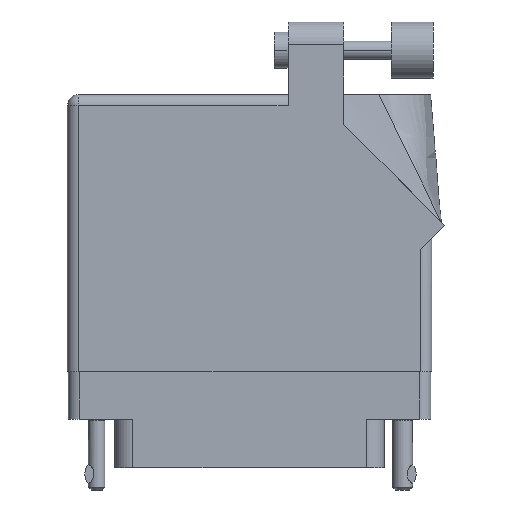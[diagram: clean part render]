
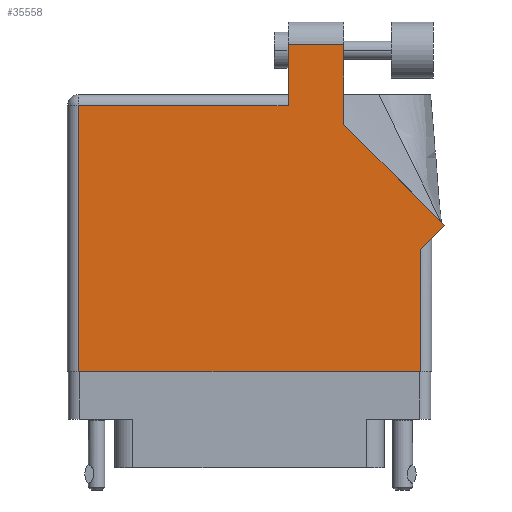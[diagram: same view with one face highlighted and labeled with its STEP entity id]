
A CAD part, front view. The second image highlights one B-rep face of the part: STEP entity #35558.
In plain terms, the highlighted face is planar.
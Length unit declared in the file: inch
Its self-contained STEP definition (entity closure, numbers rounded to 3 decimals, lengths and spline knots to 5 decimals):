
#1237 = EDGE_CURVE ( 'NONE', #14400, #40537, #26555, .T. ) ;
#1443 = CARTESIAN_POINT ( 'NONE',  ( 0., 1.468, 0. ) ) ;
#2325 = VECTOR ( 'NONE', #35104, 39.37008 ) ;
#3717 = VERTEX_POINT ( 'NONE', #31275 ) ;
#4277 = CARTESIAN_POINT ( 'NONE',  ( 1.217, 1.468, 0. ) ) ;
#5003 = EDGE_CURVE ( 'NONE', #3717, #17472, #18314, .T. ) ;
#5214 = CARTESIAN_POINT ( 'NONE',  ( 2.01, 0.737, 0. ) ) ;
#5677 = VECTOR ( 'NONE', #8949, 39.37008 ) ;
#5948 = CARTESIAN_POINT ( 'NONE',  ( 1.948, 0.737, 0. ) ) ;
#6201 = DIRECTION ( 'NONE',  ( 0., -1., 0. ) ) ;
#6716 = ORIENTED_EDGE ( 'NONE', *, *, #5003, .T. ) ;
#7235 = CARTESIAN_POINT ( 'NONE',  ( 2.08071, 0.80771, 0. ) ) ;
#8949 = DIRECTION ( 'NONE',  ( -1., 0., 0. ) ) ;
#9082 = DIRECTION ( 'NONE',  ( 1., 0., 0. ) ) ;
#9461 = ORIENTED_EDGE ( 'NONE', *, *, #38075, .T. ) ;
#9899 = VECTOR ( 'NONE', #6201, 39.37008 ) ;
#10427 = CARTESIAN_POINT ( 'NONE',  ( 0.062, 0., 0. ) ) ;
#10512 = LINE ( 'NONE', #5214, #2325 ) ;
#10582 = CARTESIAN_POINT ( 'NONE',  ( 1.524, 1.36442, 0. ) ) ;
#11581 = VERTEX_POINT ( 'NONE', #33478 ) ;
#11843 = CARTESIAN_POINT ( 'NONE',  ( 1.217, 1.805, 0. ) ) ;
#12568 = LINE ( 'NONE', #19613, #28801 ) ;
#12600 = ORIENTED_EDGE ( 'NONE', *, *, #44151, .T. ) ;
#13975 = ORIENTED_EDGE ( 'NONE', *, *, #20043, .T. ) ;
#14283 = VECTOR ( 'NONE', #41070, 39.37008 ) ;
#14400 = VERTEX_POINT ( 'NONE', #33937 ) ;
#14546 = ORIENTED_EDGE ( 'NONE', *, *, #37458, .T. ) ;
#14569 = ORIENTED_EDGE ( 'NONE', *, *, #42287, .T. ) ;
#14873 = DIRECTION ( 'NONE',  ( 0., 0., -1. ) ) ;
#15095 = LINE ( 'NONE', #24194, #9899 ) ;
#15404 = DIRECTION ( 'NONE',  ( 0., 1., 0. ) ) ;
#16024 = DIRECTION ( 'NONE',  ( -1., 0., 0. ) ) ;
#17309 = DIRECTION ( 'NONE',  ( 0., 1., 0. ) ) ;
#17425 = VECTOR ( 'NONE', #15404, 39.37008 ) ;
#17472 = VERTEX_POINT ( 'NONE', #34454 ) ;
#18314 = LINE ( 'NONE', #31293, #31669 ) ;
#19613 = CARTESIAN_POINT ( 'NONE',  ( 1.217, 1.805, 0. ) ) ;
#20043 = EDGE_CURVE ( 'NONE', #17472, #40275, #34700, .T. ) ;
#20277 = ORIENTED_EDGE ( 'NONE', *, *, #37798, .T. ) ;
#22317 = DIRECTION ( 'NONE',  ( -0.707, 0.707, 0. ) ) ;
#23098 = DIRECTION ( 'NONE',  ( -1., 0., 0. ) ) ;
#23368 = CARTESIAN_POINT ( 'NONE',  ( 1.948, 0.675, 0. ) ) ;
#23609 = VECTOR ( 'NONE', #22317, 39.37008 ) ;
#24194 = CARTESIAN_POINT ( 'NONE',  ( 1.217, 1.53, 0. ) ) ;
#25384 = VECTOR ( 'NONE', #17309, 39.37008 ) ;
#26555 = LINE ( 'NONE', #7235, #23609 ) ;
#27010 = VERTEX_POINT ( 'NONE', #11843 ) ;
#28801 = VECTOR ( 'NONE', #16024, 39.37008 ) ;
#29156 = FACE_OUTER_BOUND ( 'NONE', #36022, .T. ) ;
#29655 = CARTESIAN_POINT ( 'NONE',  ( 0., 1.53, 0. ) ) ;
#31275 = CARTESIAN_POINT ( 'NONE',  ( 0.062, 0., 0. ) ) ;
#31293 = CARTESIAN_POINT ( 'NONE',  ( 0., 0., 0. ) ) ;
#31669 = VECTOR ( 'NONE', #9082, 39.37008 ) ;
#31836 = AXIS2_PLACEMENT_3D ( 'NONE', #29655, #14873, #23098 ) ;
#32410 = LINE ( 'NONE', #1443, #5677 ) ;
#32449 = VERTEX_POINT ( 'NONE', #40043 ) ;
#33431 = CARTESIAN_POINT ( 'NONE',  ( 1.524, 1.36442, 0. ) ) ;
#33478 = CARTESIAN_POINT ( 'NONE',  ( 1.524, 1.805, 0. ) ) ;
#33937 = CARTESIAN_POINT ( 'NONE',  ( 2.08071, 0.80771, 0. ) ) ;
#34007 = LINE ( 'NONE', #10427, #14283 ) ;
#34454 = CARTESIAN_POINT ( 'NONE',  ( 1.948, 0., 0. ) ) ;
#34700 = LINE ( 'NONE', #5948, #25384 ) ;
#35104 = DIRECTION ( 'NONE',  ( 0.707, 0.707, 0. ) ) ;
#35558 = ADVANCED_FACE ( 'NONE', ( #29156 ), #44267, .F. ) ;
#36022 = EDGE_LOOP ( 'NONE', ( #20277, #38280, #9461, #14569, #12600, #6716, #13975, #14546, #42615 ) ) ;
#37458 = EDGE_CURVE ( 'NONE', #40275, #14400, #10512, .T. ) ;
#37798 = EDGE_CURVE ( 'NONE', #40537, #11581, #39505, .T. ) ;
#38075 = EDGE_CURVE ( 'NONE', #27010, #44445, #15095, .T. ) ;
#38280 = ORIENTED_EDGE ( 'NONE', *, *, #40804, .T. ) ;
#39505 = LINE ( 'NONE', #33431, #17425 ) ;
#40043 = CARTESIAN_POINT ( 'NONE',  ( 0.062, 1.468, 0. ) ) ;
#40275 = VERTEX_POINT ( 'NONE', #23368 ) ;
#40537 = VERTEX_POINT ( 'NONE', #10582 ) ;
#40804 = EDGE_CURVE ( 'NONE', #11581, #27010, #12568, .T. ) ;
#41070 = DIRECTION ( 'NONE',  ( 0., -1., 0. ) ) ;
#42287 = EDGE_CURVE ( 'NONE', #44445, #32449, #32410, .T. ) ;
#42615 = ORIENTED_EDGE ( 'NONE', *, *, #1237, .T. ) ;
#44151 = EDGE_CURVE ( 'NONE', #32449, #3717, #34007, .T. ) ;
#44267 = PLANE ( 'NONE',  #31836 ) ;
#44445 = VERTEX_POINT ( 'NONE', #4277 ) ;
